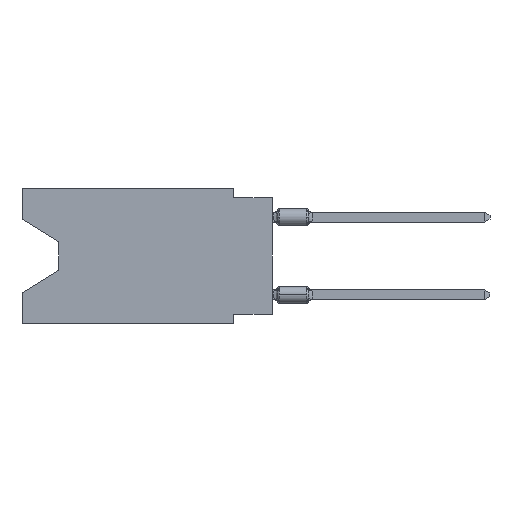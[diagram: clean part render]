
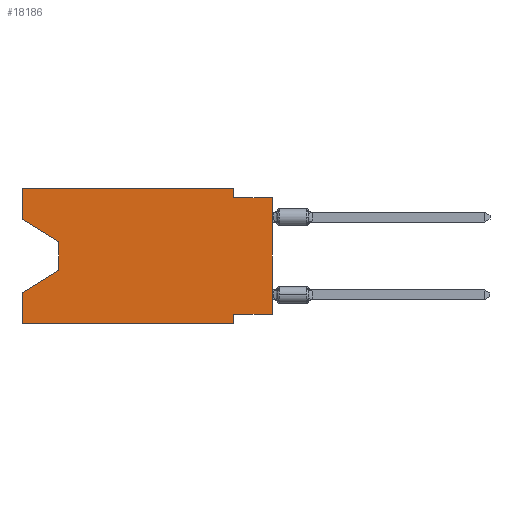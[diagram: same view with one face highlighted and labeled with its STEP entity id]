
A CAD part, left-side view. The second image highlights one B-rep face of the part: STEP entity #18186.
In plain terms, the highlighted planar face has unit normal (-1, 0, 0).
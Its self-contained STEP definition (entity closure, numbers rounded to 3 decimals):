
#125 = CARTESIAN_POINT ( 'NONE',  ( 0., 13.97, -5.385 ) ) ;
#166 = EDGE_CURVE ( 'NONE', #17954, #362, #16082, .T. ) ;
#222 = ORIENTED_EDGE ( 'NONE', *, *, #2135, .T. ) ;
#276 = LINE ( 'NONE', #15811, #2432 ) ;
#294 = VECTOR ( 'NONE', #14592, 1000. ) ;
#362 = VERTEX_POINT ( 'NONE', #2698 ) ;
#753 = CARTESIAN_POINT ( 'NONE',  ( 0., 2.54, 0. ) ) ;
#912 = EDGE_CURVE ( 'NONE', #17954, #1939, #15310, .T. ) ;
#1054 = CARTESIAN_POINT ( 'NONE',  ( 0., 2.54, -8.89 ) ) ;
#1310 = CARTESIAN_POINT ( 'NONE',  ( 0., 0., 0. ) ) ;
#1416 = LINE ( 'NONE', #15828, #2973 ) ;
#1923 = CARTESIAN_POINT ( 'NONE',  ( 0., 16.383, 0. ) ) ;
#1939 = VERTEX_POINT ( 'NONE', #6384 ) ;
#2021 = LINE ( 'NONE', #1923, #10537 ) ;
#2092 = CARTESIAN_POINT ( 'NONE',  ( 0., 2.54, -8.89 ) ) ;
#2135 = EDGE_CURVE ( 'NONE', #16104, #11867, #2762, .T. ) ;
#2161 = CARTESIAN_POINT ( 'NONE',  ( 0., 13.97, -3.505 ) ) ;
#2432 = VECTOR ( 'NONE', #5958, 1000. ) ;
#2553 = VERTEX_POINT ( 'NONE', #8049 ) ;
#2622 = DIRECTION ( 'NONE',  ( 0., -1., 0. ) ) ;
#2688 = EDGE_CURVE ( 'NONE', #14611, #3310, #1416, .T. ) ;
#2698 = CARTESIAN_POINT ( 'NONE',  ( 0., 13.97, -3.505 ) ) ;
#2762 = LINE ( 'NONE', #11305, #3901 ) ;
#2911 = CARTESIAN_POINT ( 'NONE',  ( 0., 0., -8.255 ) ) ;
#2973 = VECTOR ( 'NONE', #12854, 1000. ) ;
#3310 = VERTEX_POINT ( 'NONE', #13858 ) ;
#3318 = CARTESIAN_POINT ( 'NONE',  ( 0., 0., -0.635 ) ) ;
#3552 = LINE ( 'NONE', #2161, #10831 ) ;
#3755 = DIRECTION ( 'NONE',  ( 0., 0., -1. ) ) ;
#3901 = VECTOR ( 'NONE', #5456, 1000. ) ;
#3917 = VERTEX_POINT ( 'NONE', #3994 ) ;
#3994 = CARTESIAN_POINT ( 'NONE',  ( 0., 0., -8.255 ) ) ;
#4173 = VECTOR ( 'NONE', #2622, 1000. ) ;
#4279 = PLANE ( 'NONE',  #17353 ) ;
#4574 = ORIENTED_EDGE ( 'NONE', *, *, #10307, .T. ) ;
#4894 = DIRECTION ( 'NONE',  ( 0., -1., 0. ) ) ;
#5213 = LINE ( 'NONE', #15346, #4173 ) ;
#5338 = ORIENTED_EDGE ( 'NONE', *, *, #17718, .F. ) ;
#5456 = DIRECTION ( 'NONE',  ( 0., 0.855, -0.519 ) ) ;
#5464 = ORIENTED_EDGE ( 'NONE', *, *, #166, .T. ) ;
#5806 = VERTEX_POINT ( 'NONE', #2092 ) ;
#5958 = DIRECTION ( 'NONE',  ( 0., -1., 0. ) ) ;
#5959 = LINE ( 'NONE', #1310, #15726 ) ;
#6176 = ORIENTED_EDGE ( 'NONE', *, *, #912, .F. ) ;
#6384 = CARTESIAN_POINT ( 'NONE',  ( 0., 16.383, 0. ) ) ;
#6684 = VERTEX_POINT ( 'NONE', #8427 ) ;
#6757 = CARTESIAN_POINT ( 'NONE',  ( 0., 16.383, 0. ) ) ;
#6913 = LINE ( 'NONE', #1054, #11393 ) ;
#6980 = CARTESIAN_POINT ( 'NONE',  ( 0., 16.383, 0. ) ) ;
#7837 = DIRECTION ( 'NONE',  ( 0., 0., -1. ) ) ;
#7970 = EDGE_CURVE ( 'NONE', #6684, #11867, #2021, .T. ) ;
#8049 = CARTESIAN_POINT ( 'NONE',  ( 0., 0., -0.635 ) ) ;
#8427 = CARTESIAN_POINT ( 'NONE',  ( 0., 16.383, -8.89 ) ) ;
#9332 = ORIENTED_EDGE ( 'NONE', *, *, #2688, .F. ) ;
#10114 = ORIENTED_EDGE ( 'NONE', *, *, #13591, .F. ) ;
#10307 = EDGE_CURVE ( 'NONE', #3917, #2553, #5959, .T. ) ;
#10512 = EDGE_CURVE ( 'NONE', #1939, #14611, #5213, .T. ) ;
#10537 = VECTOR ( 'NONE', #12150, 1000. ) ;
#10831 = VECTOR ( 'NONE', #7837, 1000. ) ;
#11305 = CARTESIAN_POINT ( 'NONE',  ( 0., 13.97, -5.385 ) ) ;
#11393 = VECTOR ( 'NONE', #3755, 1000. ) ;
#11585 = EDGE_CURVE ( 'NONE', #6684, #5806, #276, .T. ) ;
#11698 = VECTOR ( 'NONE', #15640, 1000. ) ;
#11867 = VERTEX_POINT ( 'NONE', #16551 ) ;
#11938 = CARTESIAN_POINT ( 'NONE',  ( 0., 2.54, -8.255 ) ) ;
#12150 = DIRECTION ( 'NONE',  ( 0., 0., 1. ) ) ;
#12427 = DIRECTION ( 'NONE',  ( 0., 0., 1. ) ) ;
#12648 = DIRECTION ( 'NONE',  ( 0., 0., -1. ) ) ;
#12656 = DIRECTION ( 'NONE',  ( 0., 0., 1. ) ) ;
#12739 = FACE_OUTER_BOUND ( 'NONE', #16001, .T. ) ;
#12758 = LINE ( 'NONE', #2911, #11698 ) ;
#12854 = DIRECTION ( 'NONE',  ( 0., 0., -1. ) ) ;
#13074 = ORIENTED_EDGE ( 'NONE', *, *, #10512, .F. ) ;
#13591 = EDGE_CURVE ( 'NONE', #3310, #2553, #16050, .T. ) ;
#13805 = ORIENTED_EDGE ( 'NONE', *, *, #11585, .T. ) ;
#13858 = CARTESIAN_POINT ( 'NONE',  ( 0., 2.54, -0.635 ) ) ;
#14053 = VERTEX_POINT ( 'NONE', #11938 ) ;
#14416 = ORIENTED_EDGE ( 'NONE', *, *, #7970, .F. ) ;
#14592 = DIRECTION ( 'NONE',  ( 0., -0.855, -0.519 ) ) ;
#14611 = VERTEX_POINT ( 'NONE', #753 ) ;
#15310 = LINE ( 'NONE', #6757, #15452 ) ;
#15346 = CARTESIAN_POINT ( 'NONE',  ( 0., 16.383, 0. ) ) ;
#15452 = VECTOR ( 'NONE', #12427, 1000. ) ;
#15619 = DIRECTION ( 'NONE',  ( 1., 0., 0. ) ) ;
#15640 = DIRECTION ( 'NONE',  ( 0., 1., 0. ) ) ;
#15726 = VECTOR ( 'NONE', #12656, 1000. ) ;
#15746 = VECTOR ( 'NONE', #4894, 1000. ) ;
#15811 = CARTESIAN_POINT ( 'NONE',  ( 0., 16.383, -8.89 ) ) ;
#15828 = CARTESIAN_POINT ( 'NONE',  ( 0., 2.54, 0. ) ) ;
#15983 = CARTESIAN_POINT ( 'NONE',  ( 0., 16.383, -2.038 ) ) ;
#16001 = EDGE_LOOP ( 'NONE', ( #5464, #16800, #222, #14416, #13805, #16095, #5338, #4574, #10114, #9332, #13074, #6176 ) ) ;
#16050 = LINE ( 'NONE', #3318, #15746 ) ;
#16082 = LINE ( 'NONE', #15983, #294 ) ;
#16095 = ORIENTED_EDGE ( 'NONE', *, *, #17586, .F. ) ;
#16104 = VERTEX_POINT ( 'NONE', #125 ) ;
#16551 = CARTESIAN_POINT ( 'NONE',  ( 0., 16.383, -6.852 ) ) ;
#16800 = ORIENTED_EDGE ( 'NONE', *, *, #17972, .T. ) ;
#17353 = AXIS2_PLACEMENT_3D ( 'NONE', #6980, #15619, #12648 ) ;
#17404 = CARTESIAN_POINT ( 'NONE',  ( 0., 16.383, -2.038 ) ) ;
#17586 = EDGE_CURVE ( 'NONE', #14053, #5806, #6913, .T. ) ;
#17718 = EDGE_CURVE ( 'NONE', #3917, #14053, #12758, .T. ) ;
#17954 = VERTEX_POINT ( 'NONE', #17404 ) ;
#17972 = EDGE_CURVE ( 'NONE', #362, #16104, #3552, .T. ) ;
#18186 = ADVANCED_FACE ( 'NONE', ( #12739 ), #4279, .F. ) ;
